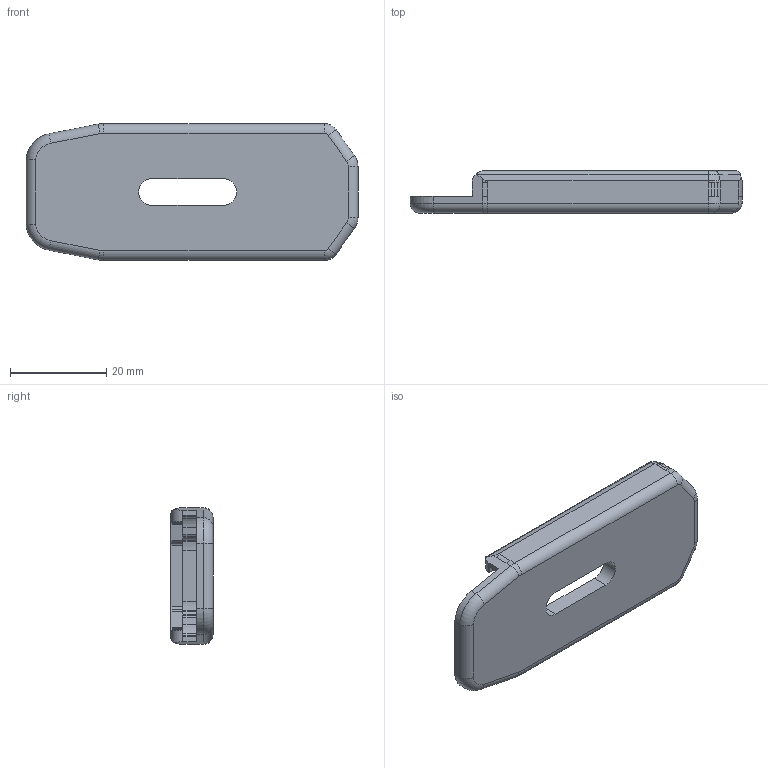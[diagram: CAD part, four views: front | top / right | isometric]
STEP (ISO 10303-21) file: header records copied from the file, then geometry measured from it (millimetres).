
FILE_DESCRIPTION (( 'STEP AP214' ), '1' );
FILE_NAME ('Base_Plate.STEP', '2022-09-24T15:52:03', ( '' ), ( '' ), 'SwSTEP 2.0', 'SolidWorks 2021', '' );
FILE_SCHEMA (( 'AUTOMOTIVE_DESIGN' ));
Length unit declared in the file: millimetre
Products named in the file (1): Base_Plate
Bounding box: 68.9 x 8.72 x 28.4 mm (x, y, z)
Volume: 7147.8 mm3; surface area: 5743.5 mm2
Topology: 1 solids, 1 shells, 126 faces, 332 edges, 208 vertices
Faces by surface type: plane 63, cylinder 45, bspline 10, torus 8
Entity records: 4576 total; most frequent: CARTESIAN_POINT 1516, ORIENTED_EDGE 664, DIRECTION 590, EDGE_CURVE 332, VERTEX_POINT 208, VECTOR 200, LINE 200, AXIS2_PLACEMENT_3D 195
